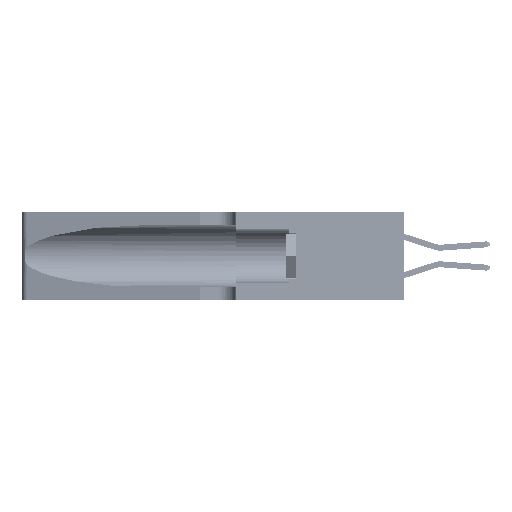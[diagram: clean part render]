
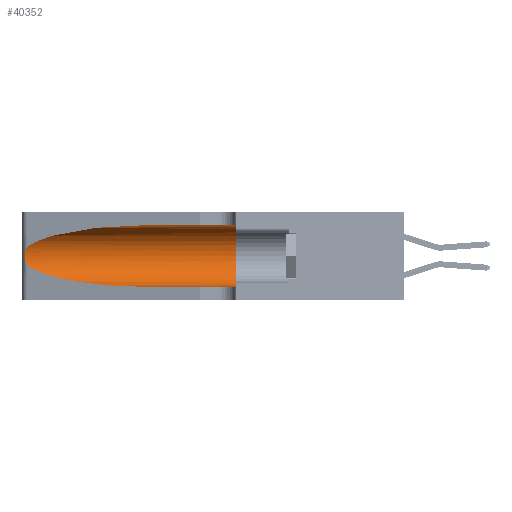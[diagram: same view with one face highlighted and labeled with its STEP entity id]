
A CAD part, left-side view. The second image highlights one B-rep face of the part: STEP entity #40352.
In plain terms, the highlighted cylindrical face has radius 3.308 mm (diameter 6.617 mm), a partial arc.
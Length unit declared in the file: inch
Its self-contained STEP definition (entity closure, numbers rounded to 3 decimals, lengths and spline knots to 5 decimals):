
#384 = ORIENTED_EDGE ( 'NONE', *, *, #14477, .F. ) ;
#397 = CARTESIAN_POINT ( 'NONE',  ( 0.25555, 1.22993, 0.14849 ) ) ;
#571 = CARTESIAN_POINT ( 'NONE',  ( 0.25639, 1.23186, 0.15144 ) ) ;
#989 = LINE ( 'NONE', #40308, #36187 ) ;
#1427 = CYLINDRICAL_SURFACE ( 'NONE', #41019, 0.13025 ) ;
#2423 = CARTESIAN_POINT ( 'NONE',  ( 0.25487, 1.22718, 0.22369 ) ) ;
#3304 = CARTESIAN_POINT ( 'NONE',  ( 0.25487, 1.22718, 0.22369 ) ) ;
#4315 = CARTESIAN_POINT ( 'NONE',  ( 0.25787, 1.23484, 0.2124 ) ) ;
#5022 = CARTESIAN_POINT ( 'NONE',  ( 0.25487, 1.22718, 0.14631 ) ) ;
#5770 = VERTEX_POINT ( 'NONE', #49298 ) ;
#5819 = CARTESIAN_POINT ( 'NONE',  ( 0.2373, 1.15595, 0.28018 ) ) ;
#7824 = CARTESIAN_POINT ( 'NONE',  ( 0.1305, 0.72297, 0.05475 ) ) ;
#9482 = VECTOR ( 'NONE', #23461, 39.37008 ) ;
#10355 = VERTEX_POINT ( 'NONE', #5022 ) ;
#10680 = LINE ( 'NONE', #16153, #9482 ) ;
#10797 = ORIENTED_EDGE ( 'NONE', *, *, #28916, .T. ) ;
#11386 = CARTESIAN_POINT ( 'NONE',  ( 0.2373, 1.15595, 0.08982 ) ) ;
#12640 = EDGE_CURVE ( 'NONE', #22155, #30090, #14573, .T. ) ;
#13572 = CARTESIAN_POINT ( 'NONE',  ( 0.1305, 1.61858, 0.185 ) ) ;
#14477 = EDGE_CURVE ( 'NONE', #33477, #5770, #46695, .T. ) ;
#14573 =( BOUNDED_CURVE ( )  B_SPLINE_CURVE ( 3, ( #33131, #37386, #5819, #2423 ),
 .UNSPECIFIED., .F., .F. ) 
 B_SPLINE_CURVE_WITH_KNOTS ( ( 4, 4 ),
 ( 1.5708, 2.84003 ),
 .UNSPECIFIED. ) 
 CURVE ( )  GEOMETRIC_REPRESENTATION_ITEM ( )  RATIONAL_B_SPLINE_CURVE ( ( 1., 0.87, 0.87, 1. ) ) 
 REPRESENTATION_ITEM ( '' )  );
#15012 = CARTESIAN_POINT ( 'NONE',  ( 0.1305, 0.72297, 0.31525 ) ) ;
#15507 = CARTESIAN_POINT ( 'NONE',  ( 0.26075, 1.23896, 0.19203 ) ) ;
#15967 = EDGE_CURVE ( 'NONE', #22155, #33477, #989, .T. ) ;
#16017 = CARTESIAN_POINT ( 'NONE',  ( 0.26017, 1.23833, 0.17102 ) ) ;
#16153 = CARTESIAN_POINT ( 'NONE',  ( 0.1305, 1.61858, 0.05475 ) ) ;
#16422 = EDGE_CURVE ( 'NONE', #10355, #26574, #32616, .T. ) ;
#18265 = ORIENTED_EDGE ( 'NONE', *, *, #36166, .T. ) ;
#20118 = CARTESIAN_POINT ( 'NONE',  ( 0.25487, 1.22718, 0.14631 ) ) ;
#20740 = DIRECTION ( 'NONE',  ( 0., -1., 0. ) ) ;
#22155 = VERTEX_POINT ( 'NONE', #15012 ) ;
#22292 = ORIENTED_EDGE ( 'NONE', *, *, #16422, .T. ) ;
#23461 = DIRECTION ( 'NONE',  ( 0., -1., 0. ) ) ;
#24006 = CARTESIAN_POINT ( 'NONE',  ( 0.25555, 1.22994, 0.2215 ) ) ;
#25346 = ORIENTED_EDGE ( 'NONE', *, *, #15967, .F. ) ;
#26574 = VERTEX_POINT ( 'NONE', #35896 ) ;
#27000 = CARTESIAN_POINT ( 'NONE',  ( 0.18966, 0.96281, 0.05475 ) ) ;
#27386 = CARTESIAN_POINT ( 'NONE',  ( 0.25856, 1.23593, 0.16098 ) ) ;
#28207 = CARTESIAN_POINT ( 'NONE',  ( 0.1305, 0.35, 0.185 ) ) ;
#28916 = EDGE_CURVE ( 'NONE', #30090, #10355, #43230, .T. ) ;
#30090 = VERTEX_POINT ( 'NONE', #33158 ) ;
#32085 = DIRECTION ( 'NONE',  ( 0., 1., 0. ) ) ;
#32616 =( BOUNDED_CURVE ( )  B_SPLINE_CURVE ( 3, ( #34630, #11386, #27000, #7824 ),
 .UNSPECIFIED., .F., .F. ) 
 B_SPLINE_CURVE_WITH_KNOTS ( ( 4, 4 ),
 ( 3.44316, 4.71239 ),
 .UNSPECIFIED. ) 
 CURVE ( )  GEOMETRIC_REPRESENTATION_ITEM ( )  RATIONAL_B_SPLINE_CURVE ( ( 1., 0.87, 0.87, 1. ) ) 
 REPRESENTATION_ITEM ( '' )  );
#33131 = CARTESIAN_POINT ( 'NONE',  ( 0.1305, 0.72297, 0.31525 ) ) ;
#33158 = CARTESIAN_POINT ( 'NONE',  ( 0.25487, 1.22718, 0.22369 ) ) ;
#33477 = VERTEX_POINT ( 'NONE', #46711 ) ;
#34630 = CARTESIAN_POINT ( 'NONE',  ( 0.25487, 1.22718, 0.14631 ) ) ;
#35225 = ORIENTED_EDGE ( 'NONE', *, *, #12640, .T. ) ;
#35500 = CARTESIAN_POINT ( 'NONE',  ( 0.25789, 1.23486, 0.15765 ) ) ;
#35896 = CARTESIAN_POINT ( 'NONE',  ( 0.1305, 0.72297, 0.05475 ) ) ;
#36151 = DIRECTION ( 'NONE',  ( 0., 0., -1. ) ) ;
#36166 = EDGE_CURVE ( 'NONE', #26574, #5770, #10680, .T. ) ;
#36187 = VECTOR ( 'NONE', #41150, 39.37008 ) ;
#36330 = DIRECTION ( 'NONE',  ( 0., 0., 1. ) ) ;
#37386 = CARTESIAN_POINT ( 'NONE',  ( 0.18966, 0.96281, 0.31525 ) ) ;
#38765 = CARTESIAN_POINT ( 'NONE',  ( 0.25639, 1.23184, 0.21858 ) ) ;
#40308 = CARTESIAN_POINT ( 'NONE',  ( 0.1305, 1.61858, 0.31525 ) ) ;
#40352 = ADVANCED_FACE ( 'NONE', ( #42141 ), #1427, .F. ) ;
#41019 = AXIS2_PLACEMENT_3D ( 'NONE', #13572, #20740, #36151 ) ;
#41150 = DIRECTION ( 'NONE',  ( 0., -1., 0. ) ) ;
#42141 = FACE_OUTER_BOUND ( 'NONE', #44956, .T. ) ;
#42672 = CARTESIAN_POINT ( 'NONE',  ( 0.26018, 1.23835, 0.19895 ) ) ;
#43230 = B_SPLINE_CURVE_WITH_KNOTS ( 'NONE', 3,
 ( #3304, #24006, #38765, #4315, #46929, #42672, #15507, #43361, #16017, #27386, #35500, #571, #397, #20118 ),
 .UNSPECIFIED., .F., .F.,
 ( 4, 2, 2, 2, 2, 2, 4 ),
 ( 0., 0.00027, 0.00053, 0.00107, 0.0016, 0.00187, 0.00214 ),
 .UNSPECIFIED. ) ;
#43361 = CARTESIAN_POINT ( 'NONE',  ( 0.26075, 1.23896, 0.178 ) ) ;
#44956 = EDGE_LOOP ( 'NONE', ( #35225, #10797, #22292, #18265, #384, #25346 ) ) ;
#46329 = AXIS2_PLACEMENT_3D ( 'NONE', #28207, #32085, #36330 ) ;
#46695 = CIRCLE ( 'NONE', #46329, 0.13025 ) ;
#46711 = CARTESIAN_POINT ( 'NONE',  ( 0.1305, 0.35, 0.31525 ) ) ;
#46929 = CARTESIAN_POINT ( 'NONE',  ( 0.25854, 1.2359, 0.20912 ) ) ;
#49298 = CARTESIAN_POINT ( 'NONE',  ( 0.1305, 0.35, 0.05475 ) ) ;
